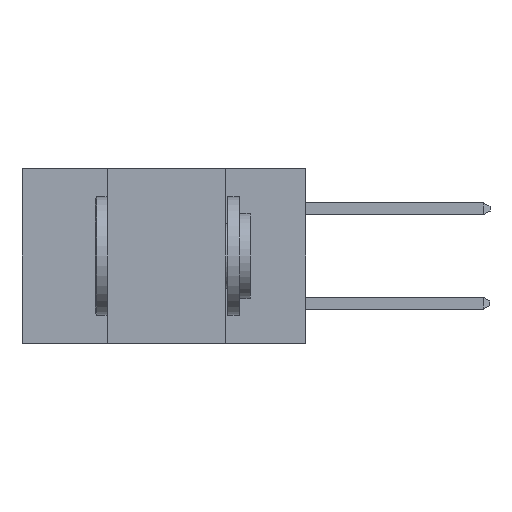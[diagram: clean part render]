
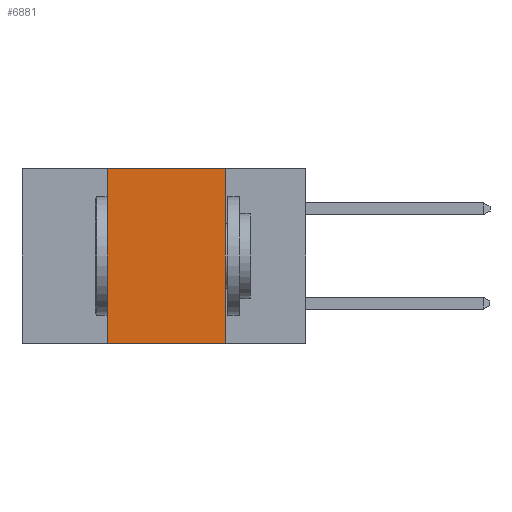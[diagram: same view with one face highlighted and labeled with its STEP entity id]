
A CAD part, left-side view. The second image highlights one B-rep face of the part: STEP entity #6881.
In plain terms, the highlighted planar face has unit normal (-1, 0, 0).
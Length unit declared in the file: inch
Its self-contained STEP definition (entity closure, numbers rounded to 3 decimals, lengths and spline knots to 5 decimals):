
#644 = VECTOR ( 'NONE', #4077, 39.37008 ) ;
#2725 = EDGE_CURVE ( 'NONE', #7420, #12375, #22729, .T. ) ;
#2744 = CARTESIAN_POINT ( 'NONE',  ( 0., 0.17, 0. ) ) ;
#3115 = ORIENTED_EDGE ( 'NONE', *, *, #2725, .F. ) ;
#3407 = LINE ( 'NONE', #7251, #14127 ) ;
#3430 = CARTESIAN_POINT ( 'NONE',  ( 0., 0.42, -0.37 ) ) ;
#3633 = DIRECTION ( 'NONE',  ( 1., 0., 0. ) ) ;
#3985 = CARTESIAN_POINT ( 'NONE',  ( 0., 0.42, 0. ) ) ;
#4077 = DIRECTION ( 'NONE',  ( 0., 0., 1. ) ) ;
#5311 = EDGE_LOOP ( 'NONE', ( #12540, #19457, #3115, #25713 ) ) ;
#5578 = DIRECTION ( 'NONE',  ( 0., -1., 0. ) ) ;
#5667 = EDGE_CURVE ( 'NONE', #22237, #24659, #9711, .T. ) ;
#6881 = ADVANCED_FACE ( 'NONE', ( #17248 ), #16445, .F. ) ;
#7251 = CARTESIAN_POINT ( 'NONE',  ( 0., 0.6, 0. ) ) ;
#7420 = VERTEX_POINT ( 'NONE', #3430 ) ;
#7591 = AXIS2_PLACEMENT_3D ( 'NONE', #14297, #3633, #18559 ) ;
#7768 = VECTOR ( 'NONE', #5578, 39.37008 ) ;
#8964 = CARTESIAN_POINT ( 'NONE',  ( 0., 0.42, 0. ) ) ;
#9711 = LINE ( 'NONE', #2744, #14668 ) ;
#12375 = VERTEX_POINT ( 'NONE', #8964 ) ;
#12511 = EDGE_CURVE ( 'NONE', #12375, #22237, #3407, .T. ) ;
#12540 = ORIENTED_EDGE ( 'NONE', *, *, #5667, .F. ) ;
#13585 = DIRECTION ( 'NONE',  ( 0., -1., 0. ) ) ;
#14127 = VECTOR ( 'NONE', #13585, 39.37008 ) ;
#14297 = CARTESIAN_POINT ( 'NONE',  ( 0., 0.6, 0. ) ) ;
#14668 = VECTOR ( 'NONE', #18864, 39.37008 ) ;
#15387 = CARTESIAN_POINT ( 'NONE',  ( 0., 0.17, -0.37 ) ) ;
#16194 = CARTESIAN_POINT ( 'NONE',  ( 0., 0.6, -0.37 ) ) ;
#16445 = PLANE ( 'NONE',  #7591 ) ;
#17248 = FACE_OUTER_BOUND ( 'NONE', #5311, .T. ) ;
#18345 = CARTESIAN_POINT ( 'NONE',  ( 0., 0.17, 0. ) ) ;
#18559 = DIRECTION ( 'NONE',  ( 0., 0., -1. ) ) ;
#18864 = DIRECTION ( 'NONE',  ( 0., 0., -1. ) ) ;
#19457 = ORIENTED_EDGE ( 'NONE', *, *, #12511, .F. ) ;
#20403 = EDGE_CURVE ( 'NONE', #7420, #24659, #24004, .T. ) ;
#22237 = VERTEX_POINT ( 'NONE', #18345 ) ;
#22729 = LINE ( 'NONE', #3985, #644 ) ;
#24004 = LINE ( 'NONE', #16194, #7768 ) ;
#24659 = VERTEX_POINT ( 'NONE', #15387 ) ;
#25713 = ORIENTED_EDGE ( 'NONE', *, *, #20403, .T. ) ;
